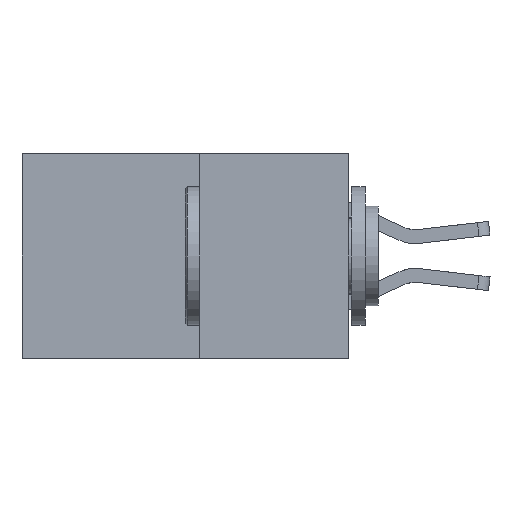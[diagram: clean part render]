
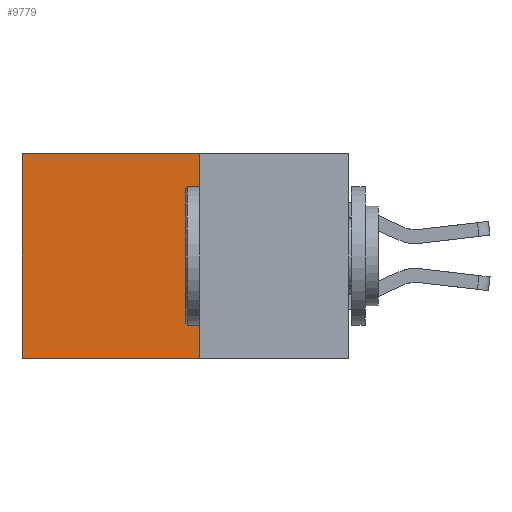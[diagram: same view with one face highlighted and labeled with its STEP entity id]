
A CAD part, left-side view. The second image highlights one B-rep face of the part: STEP entity #9779.
In plain terms, the highlighted planar face has unit normal (-1, 0, 0).
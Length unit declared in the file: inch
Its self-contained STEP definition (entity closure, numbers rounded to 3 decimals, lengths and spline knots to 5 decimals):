
#129 = DIRECTION ( 'NONE',  ( 0., 1., 0. ) ) ;
#226 = EDGE_CURVE ( 'NONE', #1607, #822, #6711, .T. ) ;
#689 = CARTESIAN_POINT ( 'NONE',  ( 0.277, 0.27, 0. ) ) ;
#822 = VERTEX_POINT ( 'NONE', #4495 ) ;
#1093 = CARTESIAN_POINT ( 'NONE',  ( 0.277, 0.27, -0.37 ) ) ;
#1522 = DIRECTION ( 'NONE',  ( 1., 0., 0. ) ) ;
#1607 = VERTEX_POINT ( 'NONE', #1093 ) ;
#1753 = EDGE_LOOP ( 'NONE', ( #9184, #7390, #3491, #5528 ) ) ;
#1898 = EDGE_CURVE ( 'NONE', #7984, #4147, #10118, .T. ) ;
#2460 = VECTOR ( 'NONE', #8071, 39.37008 ) ;
#3388 = CARTESIAN_POINT ( 'NONE',  ( 0.277, 0.59, -0.37 ) ) ;
#3491 = ORIENTED_EDGE ( 'NONE', *, *, #4745, .F. ) ;
#3788 = CARTESIAN_POINT ( 'NONE',  ( 0.277, 0.27, -0.37 ) ) ;
#4147 = VERTEX_POINT ( 'NONE', #9329 ) ;
#4408 = VECTOR ( 'NONE', #6687, 39.37008 ) ;
#4495 = CARTESIAN_POINT ( 'NONE',  ( 0.277, 0.59, -0.37 ) ) ;
#4583 = FACE_OUTER_BOUND ( 'NONE', #1753, .T. ) ;
#4584 = PLANE ( 'NONE',  #5834 ) ;
#4745 = EDGE_CURVE ( 'NONE', #7984, #1607, #6884, .T. ) ;
#4766 = VECTOR ( 'NONE', #5699, 39.37008 ) ;
#5528 = ORIENTED_EDGE ( 'NONE', *, *, #1898, .T. ) ;
#5699 = DIRECTION ( 'NONE',  ( 0., 0., -1. ) ) ;
#5834 = AXIS2_PLACEMENT_3D ( 'NONE', #6203, #1522, #6978 ) ;
#6028 = CARTESIAN_POINT ( 'NONE',  ( 0.277, 0.27, -0.37 ) ) ;
#6203 = CARTESIAN_POINT ( 'NONE',  ( 0.277, 0.27, -0.37 ) ) ;
#6481 = VECTOR ( 'NONE', #129, 39.37008 ) ;
#6687 = DIRECTION ( 'NONE',  ( 0., 1., 0. ) ) ;
#6711 = LINE ( 'NONE', #3788, #6481 ) ;
#6758 = CARTESIAN_POINT ( 'NONE',  ( 0.277, 0.27, 0. ) ) ;
#6884 = LINE ( 'NONE', #6028, #4766 ) ;
#6978 = DIRECTION ( 'NONE',  ( 0., 0., -1. ) ) ;
#6981 = EDGE_CURVE ( 'NONE', #4147, #822, #8688, .T. ) ;
#7390 = ORIENTED_EDGE ( 'NONE', *, *, #226, .F. ) ;
#7984 = VERTEX_POINT ( 'NONE', #6758 ) ;
#8071 = DIRECTION ( 'NONE',  ( 0., 0., -1. ) ) ;
#8688 = LINE ( 'NONE', #3388, #2460 ) ;
#9184 = ORIENTED_EDGE ( 'NONE', *, *, #6981, .T. ) ;
#9329 = CARTESIAN_POINT ( 'NONE',  ( 0.277, 0.59, 0. ) ) ;
#9779 = ADVANCED_FACE ( 'NONE', ( #4583 ), #4584, .F. ) ;
#10118 = LINE ( 'NONE', #689, #4408 ) ;
